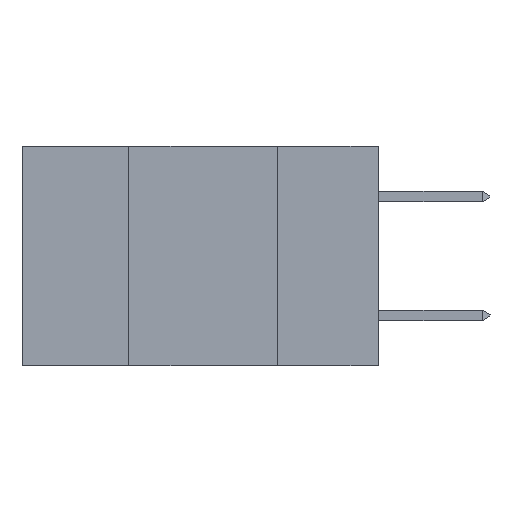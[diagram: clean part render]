
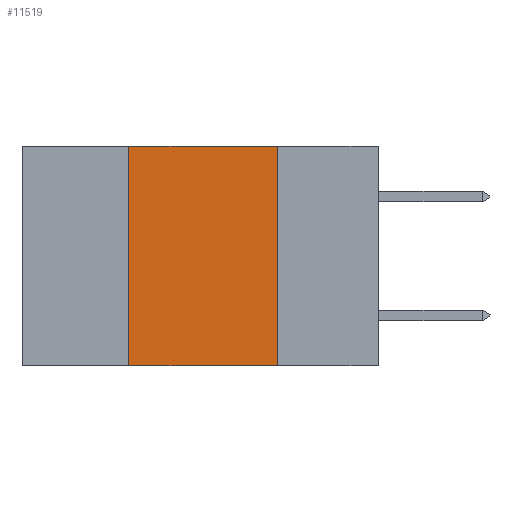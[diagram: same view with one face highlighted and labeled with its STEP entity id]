
A CAD part, left-side view. The second image highlights one B-rep face of the part: STEP entity #11519.
In plain terms, the highlighted planar face has unit normal (-1, 0, 0).
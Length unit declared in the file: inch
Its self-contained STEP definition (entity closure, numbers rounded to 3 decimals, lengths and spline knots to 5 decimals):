
#970 = DIRECTION ( 'NONE',  ( 0., 0., 1. ) ) ;
#1047 = CARTESIAN_POINT ( 'NONE',  ( 0., 0.42, 0. ) ) ;
#1439 = LINE ( 'NONE', #9413, #9542 ) ;
#1588 = LINE ( 'NONE', #1047, #2290 ) ;
#2193 = DIRECTION ( 'NONE',  ( 0., -1., 0. ) ) ;
#2290 = VECTOR ( 'NONE', #970, 39.37008 ) ;
#2447 = CARTESIAN_POINT ( 'NONE',  ( 0., 0.17, -0.37 ) ) ;
#2589 = CARTESIAN_POINT ( 'NONE',  ( 0., 0.6, 0. ) ) ;
#4057 = CARTESIAN_POINT ( 'NONE',  ( 0., 0.42, -0.37 ) ) ;
#4455 = FACE_OUTER_BOUND ( 'NONE', #4578, .T. ) ;
#4578 = EDGE_LOOP ( 'NONE', ( #18155, #4630, #6372, #5323 ) ) ;
#4630 = ORIENTED_EDGE ( 'NONE', *, *, #9117, .F. ) ;
#5323 = ORIENTED_EDGE ( 'NONE', *, *, #10730, .T. ) ;
#6372 = ORIENTED_EDGE ( 'NONE', *, *, #18376, .F. ) ;
#6825 = CARTESIAN_POINT ( 'NONE',  ( 0., 0.6, -0.37 ) ) ;
#7214 = VERTEX_POINT ( 'NONE', #4057 ) ;
#8129 = DIRECTION ( 'NONE',  ( 0., 0., -1. ) ) ;
#8408 = LINE ( 'NONE', #17762, #15765 ) ;
#9117 = EDGE_CURVE ( 'NONE', #11813, #11476, #1439, .T. ) ;
#9186 = DIRECTION ( 'NONE',  ( 0., 0., -1. ) ) ;
#9338 = VERTEX_POINT ( 'NONE', #2447 ) ;
#9413 = CARTESIAN_POINT ( 'NONE',  ( 0., 0.6, 0. ) ) ;
#9542 = VECTOR ( 'NONE', #2193, 39.37008 ) ;
#10730 = EDGE_CURVE ( 'NONE', #7214, #9338, #16326, .T. ) ;
#11105 = PLANE ( 'NONE',  #11308 ) ;
#11308 = AXIS2_PLACEMENT_3D ( 'NONE', #2589, #12627, #8129 ) ;
#11476 = VERTEX_POINT ( 'NONE', #13273 ) ;
#11519 = ADVANCED_FACE ( 'NONE', ( #4455 ), #11105, .F. ) ;
#11813 = VERTEX_POINT ( 'NONE', #17536 ) ;
#12627 = DIRECTION ( 'NONE',  ( 1., 0., 0. ) ) ;
#13273 = CARTESIAN_POINT ( 'NONE',  ( 0., 0.17, 0. ) ) ;
#14471 = EDGE_CURVE ( 'NONE', #11476, #9338, #8408, .T. ) ;
#15765 = VECTOR ( 'NONE', #9186, 39.37008 ) ;
#16326 = LINE ( 'NONE', #6825, #16772 ) ;
#16772 = VECTOR ( 'NONE', #16775, 39.37008 ) ;
#16775 = DIRECTION ( 'NONE',  ( 0., -1., 0. ) ) ;
#17536 = CARTESIAN_POINT ( 'NONE',  ( 0., 0.42, 0. ) ) ;
#17762 = CARTESIAN_POINT ( 'NONE',  ( 0., 0.17, 0. ) ) ;
#18155 = ORIENTED_EDGE ( 'NONE', *, *, #14471, .F. ) ;
#18376 = EDGE_CURVE ( 'NONE', #7214, #11813, #1588, .T. ) ;
